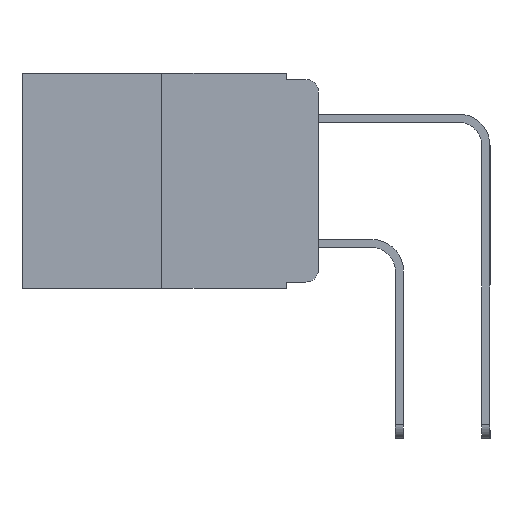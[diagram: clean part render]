
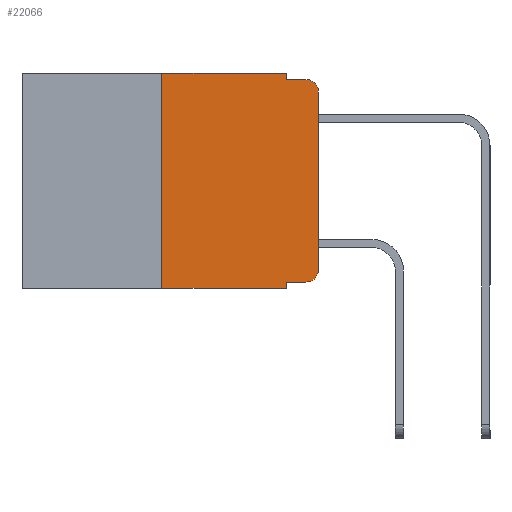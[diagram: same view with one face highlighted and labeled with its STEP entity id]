
A CAD part, left-side view. The second image highlights one B-rep face of the part: STEP entity #22066.
In plain terms, the highlighted planar face has unit normal (-1, 0, 0).
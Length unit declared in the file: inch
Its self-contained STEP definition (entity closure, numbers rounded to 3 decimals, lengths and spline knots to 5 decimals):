
#424 = VERTEX_POINT ( 'NONE', #2936 ) ;
#837 = LINE ( 'NONE', #13490, #2011 ) ;
#1131 = DIRECTION ( 'NONE',  ( 1., 0., 0. ) ) ;
#1786 = ORIENTED_EDGE ( 'NONE', *, *, #14682, .T. ) ;
#1920 = LINE ( 'NONE', #2211, #21235 ) ;
#2006 = ORIENTED_EDGE ( 'NONE', *, *, #17508, .F. ) ;
#2011 = VECTOR ( 'NONE', #15166, 39.37008 ) ;
#2211 = CARTESIAN_POINT ( 'NONE',  ( 0., 0.051, 0. ) ) ;
#2723 = LINE ( 'NONE', #14283, #12557 ) ;
#2810 = AXIS2_PLACEMENT_3D ( 'NONE', #19079, #8978, #20775 ) ;
#2930 = EDGE_CURVE ( 'NONE', #5116, #424, #14634, .T. ) ;
#2936 = CARTESIAN_POINT ( 'NONE',  ( 0., 0.051, 0. ) ) ;
#3143 = ORIENTED_EDGE ( 'NONE', *, *, #18143, .T. ) ;
#3918 = DIRECTION ( 'NONE',  ( 0., -1., 0. ) ) ;
#3973 = AXIS2_PLACEMENT_3D ( 'NONE', #9946, #1131, #13388 ) ;
#5116 = VERTEX_POINT ( 'NONE', #21041 ) ;
#5523 = CARTESIAN_POINT ( 'NONE',  ( 0., 0.051, -0.343 ) ) ;
#5852 = CARTESIAN_POINT ( 'NONE',  ( 0., 0.25, -0.343 ) ) ;
#6033 = LINE ( 'NONE', #6757, #10662 ) ;
#6380 = EDGE_LOOP ( 'NONE', ( #18636, #21842, #2006, #9452, #10546, #9737, #3143, #10021, #8678, #1786 ) ) ;
#6757 = CARTESIAN_POINT ( 'NONE',  ( 0., 0.473, -0.343 ) ) ;
#7430 = CARTESIAN_POINT ( 'NONE',  ( 0., 0.02, -0.333 ) ) ;
#8021 = CARTESIAN_POINT ( 'NONE',  ( 0., 0.25, 0. ) ) ;
#8363 = EDGE_CURVE ( 'NONE', #17190, #5116, #20250, .T. ) ;
#8449 = CARTESIAN_POINT ( 'NONE',  ( 0., 0.051, -0.01 ) ) ;
#8678 = ORIENTED_EDGE ( 'NONE', *, *, #11841, .T. ) ;
#8793 = CARTESIAN_POINT ( 'NONE',  ( 0., 0., -0.03 ) ) ;
#8929 = CARTESIAN_POINT ( 'NONE',  ( 0., 0.051, 0. ) ) ;
#8978 = DIRECTION ( 'NONE',  ( -1., 0., 0. ) ) ;
#9452 = ORIENTED_EDGE ( 'NONE', *, *, #21791, .F. ) ;
#9558 = EDGE_CURVE ( 'NONE', #9816, #15789, #837, .T. ) ;
#9737 = ORIENTED_EDGE ( 'NONE', *, *, #8363, .F. ) ;
#9816 = VERTEX_POINT ( 'NONE', #12449 ) ;
#9944 = CARTESIAN_POINT ( 'NONE',  ( 0., 0.02, -0.03 ) ) ;
#9946 = CARTESIAN_POINT ( 'NONE',  ( 0., 0.473, 0. ) ) ;
#10021 = ORIENTED_EDGE ( 'NONE', *, *, #11259, .F. ) ;
#10170 = EDGE_CURVE ( 'NONE', #15789, #15396, #11047, .T. ) ;
#10187 = DIRECTION ( 'NONE',  ( 0., -1., 0. ) ) ;
#10546 = ORIENTED_EDGE ( 'NONE', *, *, #2930, .F. ) ;
#10662 = VECTOR ( 'NONE', #20277, 39.37008 ) ;
#11047 = CIRCLE ( 'NONE', #19466, 0.02 ) ;
#11226 = VERTEX_POINT ( 'NONE', #7430 ) ;
#11259 = EDGE_CURVE ( 'NONE', #12050, #22341, #1920, .T. ) ;
#11661 = DIRECTION ( 'NONE',  ( 0., 0., -1. ) ) ;
#11841 = EDGE_CURVE ( 'NONE', #12050, #11226, #2723, .T. ) ;
#12050 = VERTEX_POINT ( 'NONE', #13183 ) ;
#12449 = CARTESIAN_POINT ( 'NONE',  ( 0., 0., -0.313 ) ) ;
#12557 = VECTOR ( 'NONE', #3918, 39.37008 ) ;
#13183 = CARTESIAN_POINT ( 'NONE',  ( 0., 0.051, -0.333 ) ) ;
#13388 = DIRECTION ( 'NONE',  ( 0., 0., -1. ) ) ;
#13490 = CARTESIAN_POINT ( 'NONE',  ( 0., 0., 0. ) ) ;
#13514 = DIRECTION ( 'NONE',  ( 0., -1., 0. ) ) ;
#14283 = CARTESIAN_POINT ( 'NONE',  ( 0., 0.051, -0.333 ) ) ;
#14442 = FACE_OUTER_BOUND ( 'NONE', #6380, .T. ) ;
#14616 = CARTESIAN_POINT ( 'NONE',  ( 0., 0.02, -0.01 ) ) ;
#14634 = LINE ( 'NONE', #15203, #18522 ) ;
#14653 = VERTEX_POINT ( 'NONE', #18934 ) ;
#14682 = EDGE_CURVE ( 'NONE', #11226, #9816, #17091, .T. ) ;
#15166 = DIRECTION ( 'NONE',  ( 0., 0., 1. ) ) ;
#15203 = CARTESIAN_POINT ( 'NONE',  ( 0., 0.473, 0. ) ) ;
#15317 = VECTOR ( 'NONE', #18135, 39.37008 ) ;
#15396 = VERTEX_POINT ( 'NONE', #14616 ) ;
#15789 = VERTEX_POINT ( 'NONE', #8793 ) ;
#17091 = CIRCLE ( 'NONE', #2810, 0.02 ) ;
#17190 = VERTEX_POINT ( 'NONE', #5852 ) ;
#17476 = VECTOR ( 'NONE', #10187, 39.37008 ) ;
#17508 = EDGE_CURVE ( 'NONE', #14653, #15396, #21974, .T. ) ;
#17625 = DIRECTION ( 'NONE',  ( 0., 0., -1. ) ) ;
#18135 = DIRECTION ( 'NONE',  ( 0., 0., 1. ) ) ;
#18143 = EDGE_CURVE ( 'NONE', #17190, #22341, #6033, .T. ) ;
#18522 = VECTOR ( 'NONE', #13514, 39.37008 ) ;
#18636 = ORIENTED_EDGE ( 'NONE', *, *, #9558, .T. ) ;
#18934 = CARTESIAN_POINT ( 'NONE',  ( 0., 0.051, -0.01 ) ) ;
#19079 = CARTESIAN_POINT ( 'NONE',  ( 0., 0.02, -0.313 ) ) ;
#19466 = AXIS2_PLACEMENT_3D ( 'NONE', #9944, #21734, #11661 ) ;
#19665 = LINE ( 'NONE', #8929, #20186 ) ;
#20002 = PLANE ( 'NONE',  #3973 ) ;
#20186 = VECTOR ( 'NONE', #21071, 39.37008 ) ;
#20250 = LINE ( 'NONE', #8021, #15317 ) ;
#20277 = DIRECTION ( 'NONE',  ( 0., -1., 0. ) ) ;
#20775 = DIRECTION ( 'NONE',  ( 0., 0., -1. ) ) ;
#21041 = CARTESIAN_POINT ( 'NONE',  ( 0., 0.25, 0. ) ) ;
#21071 = DIRECTION ( 'NONE',  ( 0., 0., -1. ) ) ;
#21235 = VECTOR ( 'NONE', #17625, 39.37008 ) ;
#21734 = DIRECTION ( 'NONE',  ( -1., 0., 0. ) ) ;
#21791 = EDGE_CURVE ( 'NONE', #424, #14653, #19665, .T. ) ;
#21842 = ORIENTED_EDGE ( 'NONE', *, *, #10170, .T. ) ;
#21974 = LINE ( 'NONE', #8449, #17476 ) ;
#22066 = ADVANCED_FACE ( 'NONE', ( #14442 ), #20002, .F. ) ;
#22341 = VERTEX_POINT ( 'NONE', #5523 ) ;
